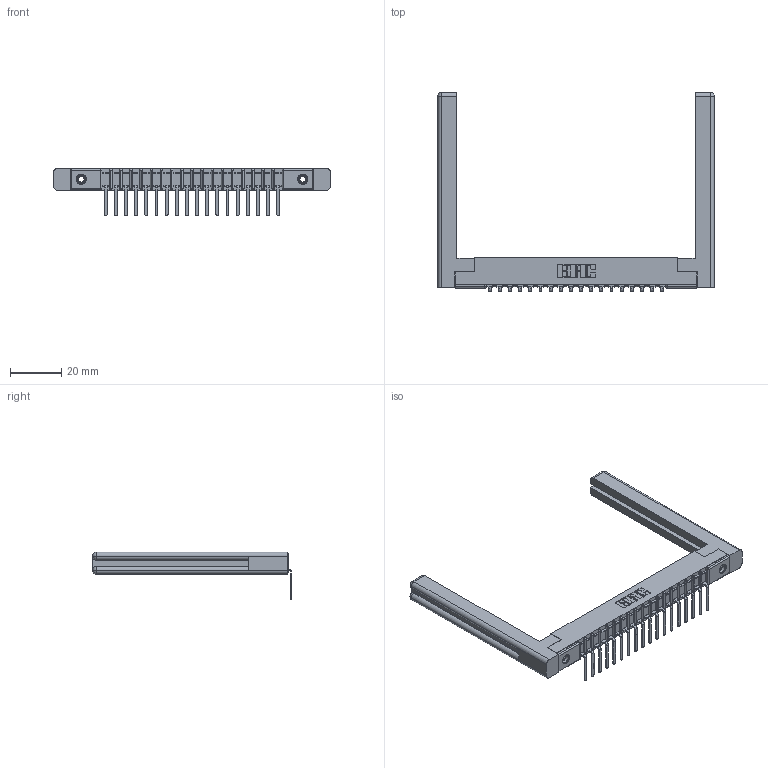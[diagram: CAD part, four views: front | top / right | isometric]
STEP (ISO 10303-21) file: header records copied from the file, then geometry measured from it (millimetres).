
FILE_DESCRIPTION (( 'STEP AP203' ), '1' );
FILE_NAME ('307-018-557-158.STEP', '2019-09-04T22:27:33', ( '' ), ( '' ), 'SwSTEP 2.0', 'SolidWorks 2016', '' );
FILE_SCHEMA (( 'CONFIG_CONTROL_DESIGN' ));
Length unit declared in the file: inch
Products named in the file (5): 307-220-058; 307-290-002_557; 307 Part_.156 Dia Mounting Holes; 307-018-557-158; 345-250-001_345-250-001-102
Assembly tree (23 placements, depth 2):
  307-018-557-158
    307 Part_.156 Dia Mounting Holes
    307-290-002_557  x18
    307-220-058  x2
    345-250-001_345-250-001-102  x2
Bounding box: 107.95 x 77.64 x 18.67 mm (x, y, z)
Volume: 14851.5 mm3; surface area: 18145.5 mm2
Topology: 23 solids, 23 shells, 1683 faces, 5069 edges, 3314 vertices
Faces by surface type: plane 1000, cylinder 621, sphere 38, torus 12, cone 12
Entity records: 21877 total; most frequent: CARTESIAN_POINT 3695, ORIENTED_EDGE 3624, DIRECTION 3562, EDGE_CURVE 1812, VECTOR 1372, LINE 1372, VERTEX_POINT 1174, AXIS2_PLACEMENT_3D 1095
